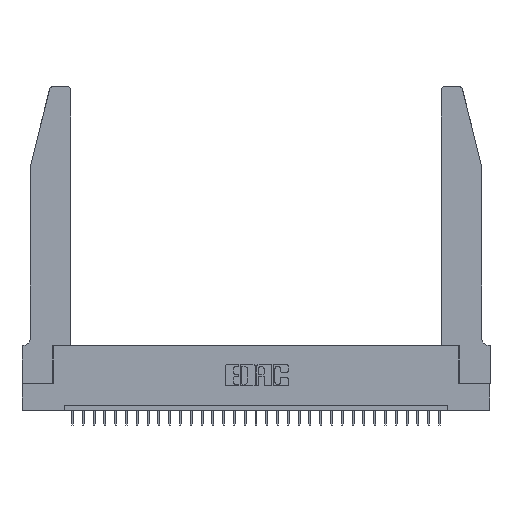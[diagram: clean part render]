
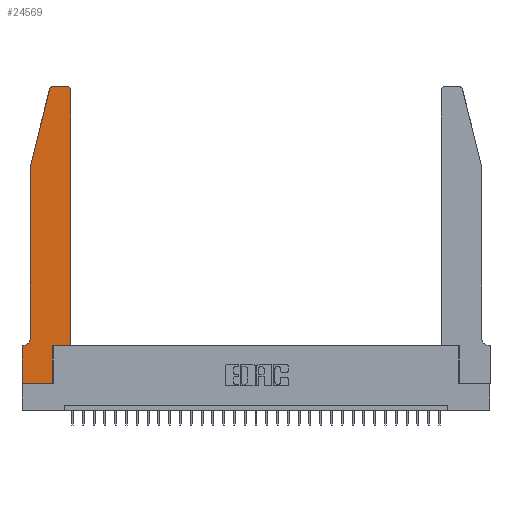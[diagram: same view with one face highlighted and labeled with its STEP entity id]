
A CAD part, top view. The second image highlights one B-rep face of the part: STEP entity #24569.
In plain terms, the highlighted planar face has unit normal (0, 0, 1).
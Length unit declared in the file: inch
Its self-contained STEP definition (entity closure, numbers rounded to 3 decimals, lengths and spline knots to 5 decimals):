
#105 = CARTESIAN_POINT ( 'NONE',  ( 0., 0.35, 0.37 ) ) ;
#253 = AXIS2_PLACEMENT_3D ( 'NONE', #24224, #2437, #19806 ) ;
#312 = LINE ( 'NONE', #10234, #31369 ) ;
#847 = EDGE_CURVE ( 'NONE', #10930, #30056, #27703, .T. ) ;
#1361 = DIRECTION ( 'NONE',  ( 1., 0., 0. ) ) ;
#2212 = ORIENTED_EDGE ( 'NONE', *, *, #14594, .T. ) ;
#2437 = DIRECTION ( 'NONE',  ( 0., 0., 1. ) ) ;
#2938 = DIRECTION ( 'NONE',  ( 1., 0., 0. ) ) ;
#3670 = ORIENTED_EDGE ( 'NONE', *, *, #6910, .T. ) ;
#3879 = VECTOR ( 'NONE', #31331, 39.37008 ) ;
#4285 = EDGE_CURVE ( 'NONE', #30056, #17963, #17561, .T. ) ;
#4595 = AXIS2_PLACEMENT_3D ( 'NONE', #16148, #23637, #1361 ) ;
#4746 = CARTESIAN_POINT ( 'NONE',  ( 0.284, 2.72, 0.37 ) ) ;
#5535 = ORIENTED_EDGE ( 'NONE', *, *, #9043, .T. ) ;
#5867 = ORIENTED_EDGE ( 'NONE', *, *, #27402, .T. ) ;
#6177 = CARTESIAN_POINT ( 'NONE',  ( 0., 0., 0.37 ) ) ;
#6362 = CARTESIAN_POINT ( 'NONE',  ( 0.0755, 0.35, 0.37 ) ) ;
#6528 = VERTEX_POINT ( 'NONE', #28112 ) ;
#6910 = EDGE_CURVE ( 'NONE', #17532, #6528, #19217, .T. ) ;
#7445 = EDGE_CURVE ( 'NONE', #18584, #17532, #31714, .T. ) ;
#7487 = FACE_OUTER_BOUND ( 'NONE', #17984, .T. ) ;
#8079 = CARTESIAN_POINT ( 'NONE',  ( 0.0755, 0.42, 0.37 ) ) ;
#8307 = LINE ( 'NONE', #6362, #8989 ) ;
#8989 = VECTOR ( 'NONE', #23101, 39.37008 ) ;
#9043 = EDGE_CURVE ( 'NONE', #13881, #22154, #23920, .T. ) ;
#9578 = ORIENTED_EDGE ( 'NONE', *, *, #17337, .T. ) ;
#9874 = VECTOR ( 'NONE', #19067, 39.37008 ) ;
#9901 = AXIS2_PLACEMENT_3D ( 'NONE', #22403, #29887, #20130 ) ;
#10234 = CARTESIAN_POINT ( 'NONE',  ( 0.2865, 0.35, 0.37 ) ) ;
#10320 = EDGE_CURVE ( 'NONE', #22154, #13523, #8307, .T. ) ;
#10410 = DIRECTION ( 'NONE',  ( 0., 0., 1. ) ) ;
#10489 = ORIENTED_EDGE ( 'NONE', *, *, #24929, .T. ) ;
#10735 = VECTOR ( 'NONE', #26219, 39.37008 ) ;
#10930 = VERTEX_POINT ( 'NONE', #19404 ) ;
#10944 = AXIS2_PLACEMENT_3D ( 'NONE', #4746, #10410, #2938 ) ;
#11902 = ORIENTED_EDGE ( 'NONE', *, *, #14462, .T. ) ;
#12006 = EDGE_CURVE ( 'NONE', #20899, #24095, #312, .T. ) ;
#12536 = CARTESIAN_POINT ( 'NONE',  ( 0.0755, 2., 0.37 ) ) ;
#12595 = DIRECTION ( 'NONE',  ( 0., 1., 0. ) ) ;
#12853 = DIRECTION ( 'NONE',  ( 0., 1., 0. ) ) ;
#13097 = CARTESIAN_POINT ( 'NONE',  ( 0., 0., 0.37 ) ) ;
#13523 = VERTEX_POINT ( 'NONE', #105 ) ;
#13813 = CARTESIAN_POINT ( 'NONE',  ( 0.4205, 2.75, 0.37 ) ) ;
#13836 = ORIENTED_EDGE ( 'NONE', *, *, #847, .T. ) ;
#13881 = VERTEX_POINT ( 'NONE', #8079 ) ;
#14462 = EDGE_CURVE ( 'NONE', #24095, #10930, #20843, .T. ) ;
#14594 = EDGE_CURVE ( 'NONE', #17963, #18584, #21805, .T. ) ;
#14650 = CARTESIAN_POINT ( 'NONE',  ( 0.4505, 2.72, 0.37 ) ) ;
#14960 = DIRECTION ( 'NONE',  ( 0., -1., 0. ) ) ;
#15045 = ORIENTED_EDGE ( 'NONE', *, *, #7445, .T. ) ;
#15084 = VECTOR ( 'NONE', #30307, 39.37008 ) ;
#15731 = CARTESIAN_POINT ( 'NONE',  ( 0.2865, 0., 0.37 ) ) ;
#16148 = CARTESIAN_POINT ( 'NONE',  ( 0.4205, 2.72, 0.37 ) ) ;
#16224 = LINE ( 'NONE', #6177, #3879 ) ;
#16464 = CARTESIAN_POINT ( 'NONE',  ( 0.2605, 2.75, 0.37 ) ) ;
#17291 = CARTESIAN_POINT ( 'NONE',  ( 0.4505, 0.35, 0.37 ) ) ;
#17337 = EDGE_CURVE ( 'NONE', #21384, #20899, #20383, .T. ) ;
#17532 = VERTEX_POINT ( 'NONE', #19494 ) ;
#17561 = CIRCLE ( 'NONE', #4595, 0.03 ) ;
#17931 = CARTESIAN_POINT ( 'NONE',  ( 0.284, 2.75, 0.37 ) ) ;
#17963 = VERTEX_POINT ( 'NONE', #13813 ) ;
#17984 = EDGE_LOOP ( 'NONE', ( #2212, #15045, #3670, #5867, #5535, #31634, #10489, #9578, #23643, #11902, #13836, #22080 ) ) ;
#18584 = VERTEX_POINT ( 'NONE', #17931 ) ;
#19067 = DIRECTION ( 'NONE',  ( -0.239, -0.971, 0. ) ) ;
#19217 = LINE ( 'NONE', #21836, #9874 ) ;
#19404 = CARTESIAN_POINT ( 'NONE',  ( 0.4505, 0.35, 0.37 ) ) ;
#19494 = CARTESIAN_POINT ( 'NONE',  ( 0.25487, 2.72718, 0.37 ) ) ;
#19806 = DIRECTION ( 'NONE',  ( 1., 0., 0. ) ) ;
#20130 = DIRECTION ( 'NONE',  ( -1., 0., 0. ) ) ;
#20383 = LINE ( 'NONE', #13097, #15084 ) ;
#20481 = VECTOR ( 'NONE', #12595, 39.37008 ) ;
#20843 = LINE ( 'NONE', #23451, #10735 ) ;
#20899 = VERTEX_POINT ( 'NONE', #15731 ) ;
#21219 = CARTESIAN_POINT ( 'NONE',  ( 0., 0., 0.37 ) ) ;
#21384 = VERTEX_POINT ( 'NONE', #21219 ) ;
#21805 = LINE ( 'NONE', #16464, #29954 ) ;
#21836 = CARTESIAN_POINT ( 'NONE',  ( 0.0755, 2., 0.37 ) ) ;
#22080 = ORIENTED_EDGE ( 'NONE', *, *, #4285, .T. ) ;
#22154 = VERTEX_POINT ( 'NONE', #25445 ) ;
#22294 = CARTESIAN_POINT ( 'NONE',  ( 0.2865, 0.35, 0.37 ) ) ;
#22403 = CARTESIAN_POINT ( 'NONE',  ( 0.0055, 0.42, 0.37 ) ) ;
#22772 = LINE ( 'NONE', #12536, #29744 ) ;
#23101 = DIRECTION ( 'NONE',  ( -1., 0., 0. ) ) ;
#23451 = CARTESIAN_POINT ( 'NONE',  ( 0.4505, 0.35, 0.37 ) ) ;
#23637 = DIRECTION ( 'NONE',  ( 0., 0., 1. ) ) ;
#23643 = ORIENTED_EDGE ( 'NONE', *, *, #12006, .T. ) ;
#23920 = CIRCLE ( 'NONE', #9901, 0.07 ) ;
#24095 = VERTEX_POINT ( 'NONE', #22294 ) ;
#24224 = CARTESIAN_POINT ( 'NONE',  ( 0., 0.35, 0.37 ) ) ;
#24569 = ADVANCED_FACE ( 'NONE', ( #7487 ), #27309, .T. ) ;
#24929 = EDGE_CURVE ( 'NONE', #13523, #21384, #16224, .T. ) ;
#25445 = CARTESIAN_POINT ( 'NONE',  ( 0.0055, 0.35, 0.37 ) ) ;
#26219 = DIRECTION ( 'NONE',  ( 1., 0., 0. ) ) ;
#27309 = PLANE ( 'NONE',  #253 ) ;
#27402 = EDGE_CURVE ( 'NONE', #6528, #13881, #22772, .T. ) ;
#27703 = LINE ( 'NONE', #17291, #20481 ) ;
#28112 = CARTESIAN_POINT ( 'NONE',  ( 0.0755, 2., 0.37 ) ) ;
#28816 = DIRECTION ( 'NONE',  ( -1., 0., 0. ) ) ;
#29744 = VECTOR ( 'NONE', #14960, 39.37008 ) ;
#29887 = DIRECTION ( 'NONE',  ( 0., 0., -1. ) ) ;
#29954 = VECTOR ( 'NONE', #28816, 39.37008 ) ;
#30056 = VERTEX_POINT ( 'NONE', #14650 ) ;
#30307 = DIRECTION ( 'NONE',  ( 1., 0., 0. ) ) ;
#31331 = DIRECTION ( 'NONE',  ( 0., -1., 0. ) ) ;
#31369 = VECTOR ( 'NONE', #12853, 39.37008 ) ;
#31634 = ORIENTED_EDGE ( 'NONE', *, *, #10320, .T. ) ;
#31714 = CIRCLE ( 'NONE', #10944, 0.03 ) ;
